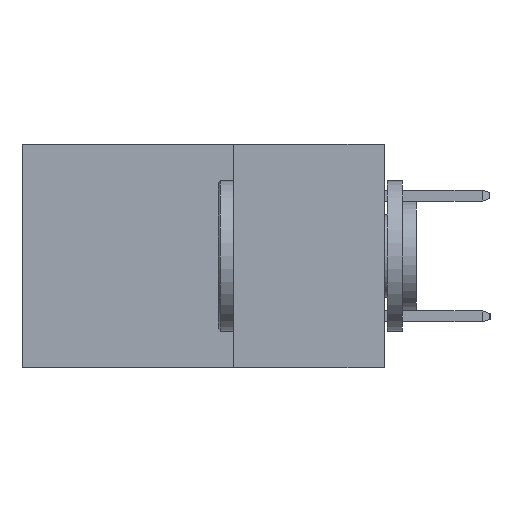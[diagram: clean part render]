
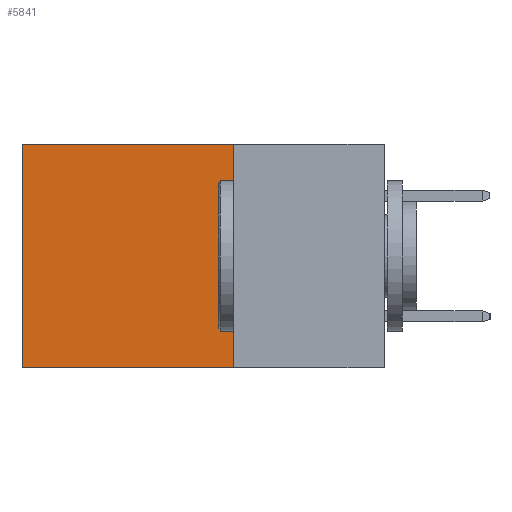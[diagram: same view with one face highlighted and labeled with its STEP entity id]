
A CAD part, left-side view. The second image highlights one B-rep face of the part: STEP entity #5841.
In plain terms, the highlighted planar face has unit normal (-1, 0, 0).
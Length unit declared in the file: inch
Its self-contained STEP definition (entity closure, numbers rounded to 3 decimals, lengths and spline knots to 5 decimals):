
#56 = DIRECTION ( 'NONE',  ( 1., 0., 0. ) ) ;
#162 = LINE ( 'NONE', #7571, #3948 ) ;
#188 = PLANE ( 'NONE',  #7680 ) ;
#349 = DIRECTION ( 'NONE',  ( 0., 0., -1. ) ) ;
#657 = DIRECTION ( 'NONE',  ( 0., 0., -1. ) ) ;
#714 = VERTEX_POINT ( 'NONE', #3757 ) ;
#1063 = EDGE_CURVE ( 'NONE', #5640, #4457, #7487, .T. ) ;
#1679 = CARTESIAN_POINT ( 'NONE',  ( 0.2615, 0.6, 0. ) ) ;
#1700 = VECTOR ( 'NONE', #5615, 39.37008 ) ;
#1923 = ORIENTED_EDGE ( 'NONE', *, *, #1063, .T. ) ;
#2601 = ORIENTED_EDGE ( 'NONE', *, *, #4969, .F. ) ;
#2629 = VECTOR ( 'NONE', #6407, 39.37008 ) ;
#2737 = ORIENTED_EDGE ( 'NONE', *, *, #3614, .F. ) ;
#2839 = ORIENTED_EDGE ( 'NONE', *, *, #6806, .T. ) ;
#3614 = EDGE_CURVE ( 'NONE', #6140, #714, #4791, .T. ) ;
#3757 = CARTESIAN_POINT ( 'NONE',  ( 0.2615, 0.25, -0.37 ) ) ;
#3948 = VECTOR ( 'NONE', #7539, 39.37008 ) ;
#4243 = CARTESIAN_POINT ( 'NONE',  ( 0.2615, 0.6, -0.37 ) ) ;
#4457 = VERTEX_POINT ( 'NONE', #7828 ) ;
#4791 = LINE ( 'NONE', #6437, #2629 ) ;
#4969 = EDGE_CURVE ( 'NONE', #714, #4457, #5802, .T. ) ;
#5615 = DIRECTION ( 'NONE',  ( 0., 1., 0. ) ) ;
#5640 = VERTEX_POINT ( 'NONE', #1679 ) ;
#5802 = LINE ( 'NONE', #5876, #1700 ) ;
#5841 = ADVANCED_FACE ( 'NONE', ( #6740 ), #188, .F. ) ;
#5876 = CARTESIAN_POINT ( 'NONE',  ( 0.2615, 0.25, -0.37 ) ) ;
#6140 = VERTEX_POINT ( 'NONE', #7818 ) ;
#6407 = DIRECTION ( 'NONE',  ( 0., 0., -1. ) ) ;
#6437 = CARTESIAN_POINT ( 'NONE',  ( 0.2615, 0.25, -0.37 ) ) ;
#6740 = FACE_OUTER_BOUND ( 'NONE', #8189, .T. ) ;
#6806 = EDGE_CURVE ( 'NONE', #6140, #5640, #162, .T. ) ;
#7487 = LINE ( 'NONE', #4243, #9017 ) ;
#7539 = DIRECTION ( 'NONE',  ( 0., 1., 0. ) ) ;
#7571 = CARTESIAN_POINT ( 'NONE',  ( 0.2615, 0.25, 0. ) ) ;
#7680 = AXIS2_PLACEMENT_3D ( 'NONE', #8874, #56, #349 ) ;
#7818 = CARTESIAN_POINT ( 'NONE',  ( 0.2615, 0.25, 0. ) ) ;
#7828 = CARTESIAN_POINT ( 'NONE',  ( 0.2615, 0.6, -0.37 ) ) ;
#8189 = EDGE_LOOP ( 'NONE', ( #1923, #2601, #2737, #2839 ) ) ;
#8874 = CARTESIAN_POINT ( 'NONE',  ( 0.2615, 0.25, -0.37 ) ) ;
#9017 = VECTOR ( 'NONE', #657, 39.37008 ) ;
